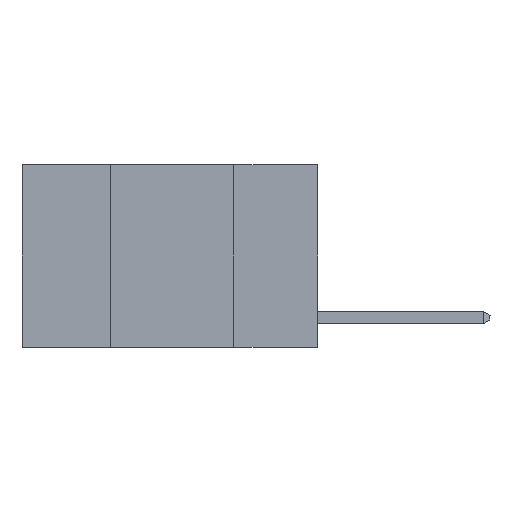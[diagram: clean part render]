
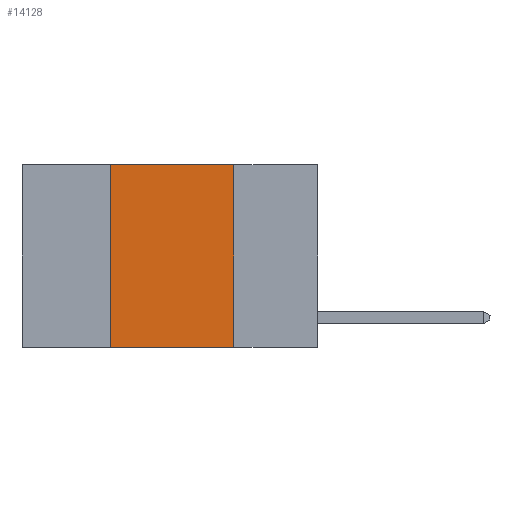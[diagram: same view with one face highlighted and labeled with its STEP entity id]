
A CAD part, left-side view. The second image highlights one B-rep face of the part: STEP entity #14128.
In plain terms, the highlighted planar face has unit normal (-1, 0, 0).
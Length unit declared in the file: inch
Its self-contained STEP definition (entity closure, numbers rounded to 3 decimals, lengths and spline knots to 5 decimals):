
#1276 = CARTESIAN_POINT ( 'NONE',  ( 0., 0.6, 0. ) ) ;
#2305 = EDGE_CURVE ( 'NONE', #7116, #6141, #10846, .T. ) ;
#3598 = DIRECTION ( 'NONE',  ( 1., 0., 0. ) ) ;
#5192 = VERTEX_POINT ( 'NONE', #16097 ) ;
#6141 = VERTEX_POINT ( 'NONE', #8248 ) ;
#7116 = VERTEX_POINT ( 'NONE', #18687 ) ;
#8248 = CARTESIAN_POINT ( 'NONE',  ( 0., 0.42, 0. ) ) ;
#8494 = VECTOR ( 'NONE', #15490, 39.37008 ) ;
#9220 = LINE ( 'NONE', #13186, #8494 ) ;
#9700 = CARTESIAN_POINT ( 'NONE',  ( 0., 0.6, 0. ) ) ;
#10346 = FACE_OUTER_BOUND ( 'NONE', #29419, .T. ) ;
#10846 = LINE ( 'NONE', #26769, #22918 ) ;
#10898 = DIRECTION ( 'NONE',  ( 0., 0., 1. ) ) ;
#11671 = VECTOR ( 'NONE', #25542, 39.37008 ) ;
#12670 = VECTOR ( 'NONE', #22446, 39.37008 ) ;
#13186 = CARTESIAN_POINT ( 'NONE',  ( 0., 0.6, -0.37 ) ) ;
#13716 = ORIENTED_EDGE ( 'NONE', *, *, #2305, .F. ) ;
#14128 = ADVANCED_FACE ( 'NONE', ( #10346 ), #15080, .F. ) ;
#15080 = PLANE ( 'NONE',  #23879 ) ;
#15235 = EDGE_CURVE ( 'NONE', #7116, #18903, #9220, .T. ) ;
#15490 = DIRECTION ( 'NONE',  ( 0., -1., 0. ) ) ;
#16097 = CARTESIAN_POINT ( 'NONE',  ( 0., 0.17, 0. ) ) ;
#16345 = LINE ( 'NONE', #9700, #11671 ) ;
#17417 = EDGE_CURVE ( 'NONE', #6141, #5192, #16345, .T. ) ;
#18687 = CARTESIAN_POINT ( 'NONE',  ( 0., 0.42, -0.37 ) ) ;
#18903 = VERTEX_POINT ( 'NONE', #23638 ) ;
#19676 = DIRECTION ( 'NONE',  ( 0., 0., -1. ) ) ;
#20203 = CARTESIAN_POINT ( 'NONE',  ( 0., 0.17, 0. ) ) ;
#22446 = DIRECTION ( 'NONE',  ( 0., 0., -1. ) ) ;
#22597 = ORIENTED_EDGE ( 'NONE', *, *, #17417, .F. ) ;
#22819 = EDGE_CURVE ( 'NONE', #5192, #18903, #24736, .T. ) ;
#22918 = VECTOR ( 'NONE', #10898, 39.37008 ) ;
#23638 = CARTESIAN_POINT ( 'NONE',  ( 0., 0.17, -0.37 ) ) ;
#23879 = AXIS2_PLACEMENT_3D ( 'NONE', #1276, #3598, #19676 ) ;
#23994 = ORIENTED_EDGE ( 'NONE', *, *, #22819, .F. ) ;
#24736 = LINE ( 'NONE', #20203, #12670 ) ;
#25469 = ORIENTED_EDGE ( 'NONE', *, *, #15235, .T. ) ;
#25542 = DIRECTION ( 'NONE',  ( 0., -1., 0. ) ) ;
#26769 = CARTESIAN_POINT ( 'NONE',  ( 0., 0.42, 0. ) ) ;
#29419 = EDGE_LOOP ( 'NONE', ( #23994, #22597, #13716, #25469 ) ) ;
